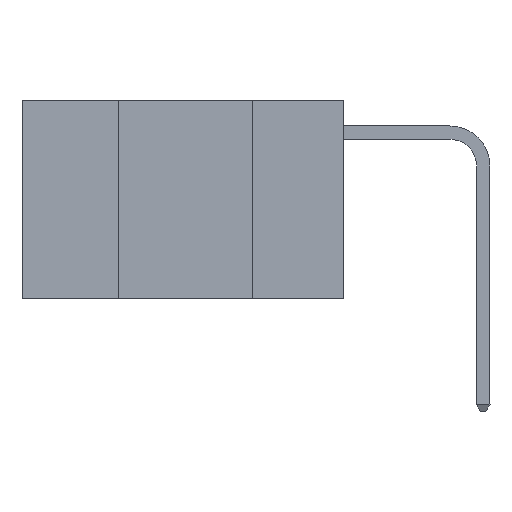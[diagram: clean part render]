
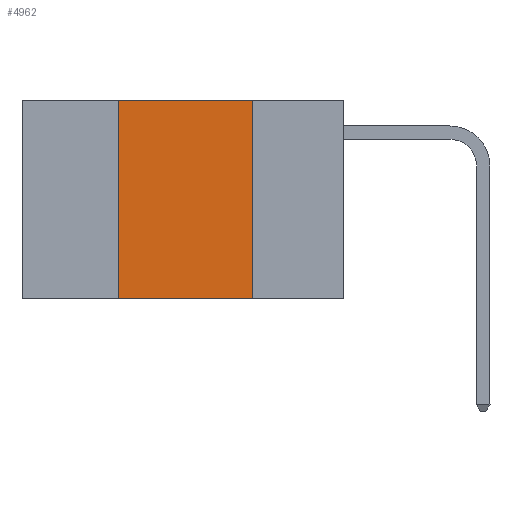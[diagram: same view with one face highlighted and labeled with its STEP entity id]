
A CAD part, left-side view. The second image highlights one B-rep face of the part: STEP entity #4962.
In plain terms, the highlighted planar face has unit normal (-1, 0, 0).
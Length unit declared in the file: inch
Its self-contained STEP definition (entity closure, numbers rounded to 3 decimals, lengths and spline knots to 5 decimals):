
#579 = EDGE_CURVE ( 'NONE', #3196, #3880, #1643, .T. ) ;
#1643 = LINE ( 'NONE', #6735, #16192 ) ;
#1752 = CARTESIAN_POINT ( 'NONE',  ( 0., 0.17, 0. ) ) ;
#1780 = ORIENTED_EDGE ( 'NONE', *, *, #15596, .F. ) ;
#1781 = CARTESIAN_POINT ( 'NONE',  ( 0., 0.42, -0.37 ) ) ;
#2298 = EDGE_LOOP ( 'NONE', ( #1780, #14774, #16364, #14146 ) ) ;
#3068 = DIRECTION ( 'NONE',  ( 0., -1., 0. ) ) ;
#3196 = VERTEX_POINT ( 'NONE', #1781 ) ;
#3880 = VERTEX_POINT ( 'NONE', #15081 ) ;
#3966 = EDGE_CURVE ( 'NONE', #3196, #6029, #15486, .T. ) ;
#3978 = CARTESIAN_POINT ( 'NONE',  ( 0., 0.6, -0.37 ) ) ;
#4115 = FACE_OUTER_BOUND ( 'NONE', #2298, .T. ) ;
#4149 = VECTOR ( 'NONE', #3068, 39.37008 ) ;
#4962 = ADVANCED_FACE ( 'NONE', ( #4115 ), #10275, .F. ) ;
#5247 = DIRECTION ( 'NONE',  ( 0., -1., 0. ) ) ;
#5963 = LINE ( 'NONE', #1752, #6669 ) ;
#6029 = VERTEX_POINT ( 'NONE', #9957 ) ;
#6669 = VECTOR ( 'NONE', #9497, 39.37008 ) ;
#6703 = CARTESIAN_POINT ( 'NONE',  ( 0., 0.6, 0. ) ) ;
#6735 = CARTESIAN_POINT ( 'NONE',  ( 0., 0.42, 0. ) ) ;
#6756 = AXIS2_PLACEMENT_3D ( 'NONE', #6703, #9016, #9428 ) ;
#8773 = CARTESIAN_POINT ( 'NONE',  ( 0., 0.17, 0. ) ) ;
#9016 = DIRECTION ( 'NONE',  ( 1., 0., 0. ) ) ;
#9428 = DIRECTION ( 'NONE',  ( 0., 0., -1. ) ) ;
#9497 = DIRECTION ( 'NONE',  ( 0., 0., -1. ) ) ;
#9957 = CARTESIAN_POINT ( 'NONE',  ( 0., 0.17, -0.37 ) ) ;
#9999 = LINE ( 'NONE', #15094, #16469 ) ;
#10275 = PLANE ( 'NONE',  #6756 ) ;
#11893 = EDGE_CURVE ( 'NONE', #3880, #14445, #9999, .T. ) ;
#13143 = DIRECTION ( 'NONE',  ( 0., 0., 1. ) ) ;
#14146 = ORIENTED_EDGE ( 'NONE', *, *, #3966, .T. ) ;
#14445 = VERTEX_POINT ( 'NONE', #8773 ) ;
#14774 = ORIENTED_EDGE ( 'NONE', *, *, #11893, .F. ) ;
#15081 = CARTESIAN_POINT ( 'NONE',  ( 0., 0.42, 0. ) ) ;
#15094 = CARTESIAN_POINT ( 'NONE',  ( 0., 0.6, 0. ) ) ;
#15486 = LINE ( 'NONE', #3978, #4149 ) ;
#15596 = EDGE_CURVE ( 'NONE', #14445, #6029, #5963, .T. ) ;
#16192 = VECTOR ( 'NONE', #13143, 39.37008 ) ;
#16364 = ORIENTED_EDGE ( 'NONE', *, *, #579, .F. ) ;
#16469 = VECTOR ( 'NONE', #5247, 39.37008 ) ;
